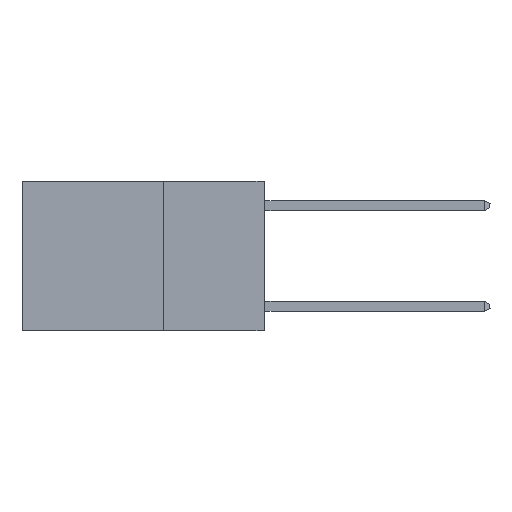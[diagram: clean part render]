
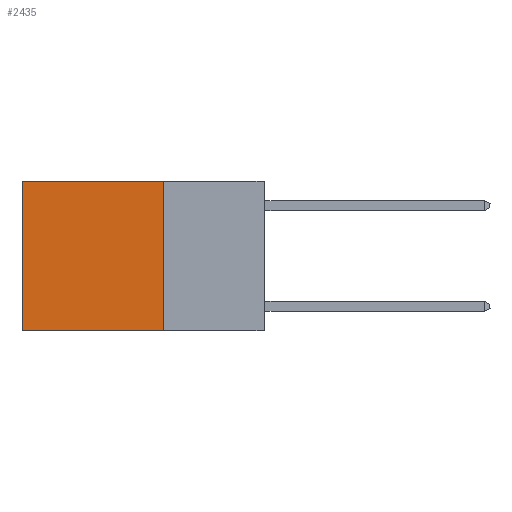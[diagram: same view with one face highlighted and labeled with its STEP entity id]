
A CAD part, left-side view. The second image highlights one B-rep face of the part: STEP entity #2435.
In plain terms, the highlighted planar face has unit normal (-1, 0, 0).
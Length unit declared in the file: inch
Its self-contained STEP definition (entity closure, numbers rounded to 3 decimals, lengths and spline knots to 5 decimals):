
#605 = DIRECTION ( 'NONE',  ( 0., 0., -1. ) ) ;
#1740 = LINE ( 'NONE', #13443, #11196 ) ;
#1784 = EDGE_LOOP ( 'NONE', ( #9249, #8751, #16413, #11438 ) ) ;
#2104 = CARTESIAN_POINT ( 'NONE',  ( 0.2625, 0.25, 0. ) ) ;
#2435 = ADVANCED_FACE ( 'NONE', ( #7162 ), #8561, .F. ) ;
#2696 = CARTESIAN_POINT ( 'NONE',  ( 0.2625, 0.25, 0. ) ) ;
#2700 = VERTEX_POINT ( 'NONE', #14175 ) ;
#2996 = EDGE_CURVE ( 'NONE', #9070, #10227, #17027, .T. ) ;
#3672 = DIRECTION ( 'NONE',  ( 0., 1., 0. ) ) ;
#4193 = CARTESIAN_POINT ( 'NONE',  ( 0.2625, 0.25, -0.37 ) ) ;
#5921 = DIRECTION ( 'NONE',  ( 1., 0., 0. ) ) ;
#6555 = VECTOR ( 'NONE', #7615, 39.37008 ) ;
#7162 = FACE_OUTER_BOUND ( 'NONE', #1784, .T. ) ;
#7476 = AXIS2_PLACEMENT_3D ( 'NONE', #13174, #5921, #11392 ) ;
#7615 = DIRECTION ( 'NONE',  ( 0., 0., -1. ) ) ;
#8329 = CARTESIAN_POINT ( 'NONE',  ( 0.2625, 0.6, -0.37 ) ) ;
#8411 = CARTESIAN_POINT ( 'NONE',  ( 0.2625, 0.25, -0.37 ) ) ;
#8561 = PLANE ( 'NONE',  #7476 ) ;
#8751 = ORIENTED_EDGE ( 'NONE', *, *, #2996, .F. ) ;
#9067 = EDGE_CURVE ( 'NONE', #2700, #10382, #12709, .T. ) ;
#9070 = VERTEX_POINT ( 'NONE', #4193 ) ;
#9249 = ORIENTED_EDGE ( 'NONE', *, *, #11000, .T. ) ;
#10227 = VERTEX_POINT ( 'NONE', #8329 ) ;
#10382 = VERTEX_POINT ( 'NONE', #18487 ) ;
#11000 = EDGE_CURVE ( 'NONE', #10382, #10227, #1740, .T. ) ;
#11196 = VECTOR ( 'NONE', #605, 39.37008 ) ;
#11392 = DIRECTION ( 'NONE',  ( 0., 0., -1. ) ) ;
#11438 = ORIENTED_EDGE ( 'NONE', *, *, #9067, .T. ) ;
#11654 = LINE ( 'NONE', #2104, #6555 ) ;
#12151 = EDGE_CURVE ( 'NONE', #2700, #9070, #11654, .T. ) ;
#12709 = LINE ( 'NONE', #2696, #12775 ) ;
#12775 = VECTOR ( 'NONE', #3672, 39.37008 ) ;
#13174 = CARTESIAN_POINT ( 'NONE',  ( 0.2625, 0.25, 0. ) ) ;
#13443 = CARTESIAN_POINT ( 'NONE',  ( 0.2625, 0.6, 0. ) ) ;
#14175 = CARTESIAN_POINT ( 'NONE',  ( 0.2625, 0.25, 0. ) ) ;
#14409 = DIRECTION ( 'NONE',  ( 0., 1., 0. ) ) ;
#16413 = ORIENTED_EDGE ( 'NONE', *, *, #12151, .F. ) ;
#17027 = LINE ( 'NONE', #8411, #17552 ) ;
#17552 = VECTOR ( 'NONE', #14409, 39.37008 ) ;
#18487 = CARTESIAN_POINT ( 'NONE',  ( 0.2625, 0.6, 0. ) ) ;
